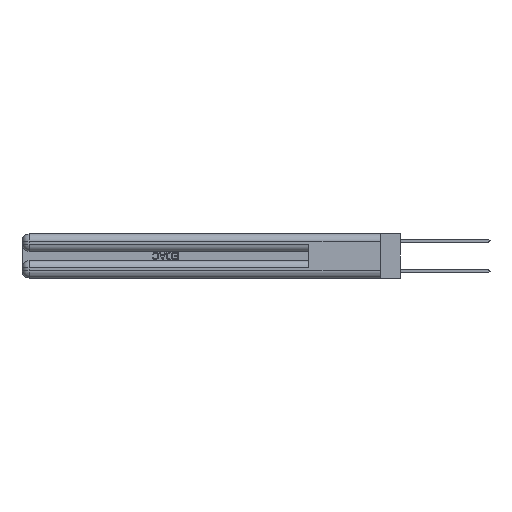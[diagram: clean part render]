
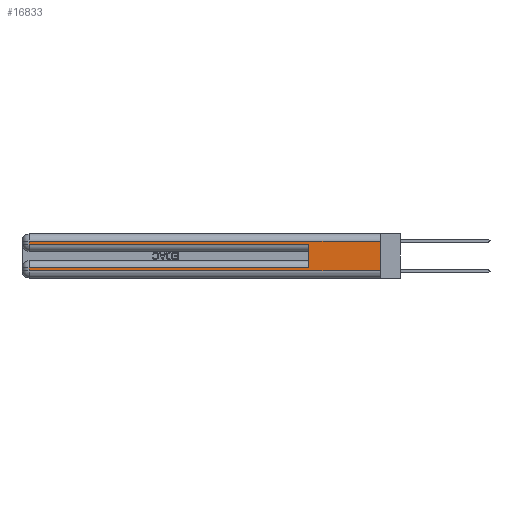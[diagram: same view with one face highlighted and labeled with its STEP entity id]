
A CAD part, left-side view. The second image highlights one B-rep face of the part: STEP entity #16833.
In plain terms, the highlighted planar face has unit normal (-1, 0, 0).
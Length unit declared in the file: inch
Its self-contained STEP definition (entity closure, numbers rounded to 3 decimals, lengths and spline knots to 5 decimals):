
#198 = EDGE_CURVE ( 'NONE', #7042, #27599, #11728, .T. ) ;
#720 = ORIENTED_EDGE ( 'NONE', *, *, #17180, .F. ) ;
#1212 = CARTESIAN_POINT ( 'NONE',  ( 0., 0.6, 0.285 ) ) ;
#1378 = CARTESIAN_POINT ( 'NONE',  ( 0., 0., 0.285 ) ) ;
#2588 = ORIENTED_EDGE ( 'NONE', *, *, #14866, .T. ) ;
#3160 = ORIENTED_EDGE ( 'NONE', *, *, #25296, .F. ) ;
#3190 = CARTESIAN_POINT ( 'NONE',  ( 0., 0., 0.37 ) ) ;
#4592 = EDGE_CURVE ( 'NONE', #10949, #34986, #30109, .T. ) ;
#5843 = CARTESIAN_POINT ( 'NONE',  ( 0., 0., 0.06 ) ) ;
#5926 = DIRECTION ( 'NONE',  ( 0., 0., 1. ) ) ;
#6477 = CARTESIAN_POINT ( 'NONE',  ( 0., 0., 0.31 ) ) ;
#6517 = FACE_OUTER_BOUND ( 'NONE', #27968, .T. ) ;
#7042 = VERTEX_POINT ( 'NONE', #21758 ) ;
#7309 = CARTESIAN_POINT ( 'NONE',  ( 0., 2.94, 0.06 ) ) ;
#7376 = VERTEX_POINT ( 'NONE', #7309 ) ;
#7793 = DIRECTION ( 'NONE',  ( 0., 0., -1. ) ) ;
#7991 = CARTESIAN_POINT ( 'NONE',  ( 0., 0., 0.37 ) ) ;
#8673 = LINE ( 'NONE', #25669, #31384 ) ;
#9065 = CARTESIAN_POINT ( 'NONE',  ( 0., 2.94, 0.085 ) ) ;
#10949 = VERTEX_POINT ( 'NONE', #22416 ) ;
#11449 = LINE ( 'NONE', #5843, #21288 ) ;
#11728 = LINE ( 'NONE', #6477, #22812 ) ;
#11773 = PLANE ( 'NONE',  #25921 ) ;
#11873 = VECTOR ( 'NONE', #5926, 39.37008 ) ;
#13426 = LINE ( 'NONE', #7991, #13972 ) ;
#13459 = EDGE_CURVE ( 'NONE', #27599, #10949, #15153, .T. ) ;
#13959 = LINE ( 'NONE', #25172, #11873 ) ;
#13972 = VECTOR ( 'NONE', #7793, 39.37008 ) ;
#14409 = VERTEX_POINT ( 'NONE', #9065 ) ;
#14560 = DIRECTION ( 'NONE',  ( 1., 0., 0. ) ) ;
#14866 = EDGE_CURVE ( 'NONE', #14409, #7376, #17289, .T. ) ;
#15142 = CARTESIAN_POINT ( 'NONE',  ( 0., 2.94, 0.31 ) ) ;
#15153 = LINE ( 'NONE', #35053, #28697 ) ;
#15573 = CARTESIAN_POINT ( 'NONE',  ( 0., 0., 0.06 ) ) ;
#16241 = ORIENTED_EDGE ( 'NONE', *, *, #13459, .T. ) ;
#16833 = ADVANCED_FACE ( 'NONE', ( #6517 ), #11773, .F. ) ;
#17180 = EDGE_CURVE ( 'NONE', #7042, #26058, #13426, .T. ) ;
#17289 = LINE ( 'NONE', #28630, #29357 ) ;
#19382 = VERTEX_POINT ( 'NONE', #27951 ) ;
#21129 = DIRECTION ( 'NONE',  ( 0., 0., -1. ) ) ;
#21272 = EDGE_CURVE ( 'NONE', #19382, #14409, #8673, .T. ) ;
#21288 = VECTOR ( 'NONE', #34528, 39.37008 ) ;
#21702 = EDGE_CURVE ( 'NONE', #7376, #26058, #11449, .T. ) ;
#21758 = CARTESIAN_POINT ( 'NONE',  ( 0., 0., 0.31 ) ) ;
#22330 = ORIENTED_EDGE ( 'NONE', *, *, #4592, .T. ) ;
#22416 = CARTESIAN_POINT ( 'NONE',  ( 0., 2.94, 0.285 ) ) ;
#22812 = VECTOR ( 'NONE', #34435, 39.37008 ) ;
#24025 = ORIENTED_EDGE ( 'NONE', *, *, #198, .T. ) ;
#25172 = CARTESIAN_POINT ( 'NONE',  ( 0., 0.6, 0.145 ) ) ;
#25296 = EDGE_CURVE ( 'NONE', #19382, #34986, #13959, .T. ) ;
#25669 = CARTESIAN_POINT ( 'NONE',  ( 0., 0., 0.085 ) ) ;
#25921 = AXIS2_PLACEMENT_3D ( 'NONE', #3190, #14560, #28913 ) ;
#26058 = VERTEX_POINT ( 'NONE', #15573 ) ;
#26941 = DIRECTION ( 'NONE',  ( 0., -1., 0. ) ) ;
#27599 = VERTEX_POINT ( 'NONE', #15142 ) ;
#27951 = CARTESIAN_POINT ( 'NONE',  ( 0., 0.6, 0.085 ) ) ;
#27968 = EDGE_LOOP ( 'NONE', ( #720, #24025, #16241, #22330, #3160, #36279, #2588, #36660 ) ) ;
#28614 = VECTOR ( 'NONE', #26941, 39.37008 ) ;
#28630 = CARTESIAN_POINT ( 'NONE',  ( 0., 2.94, 0.37 ) ) ;
#28697 = VECTOR ( 'NONE', #21129, 39.37008 ) ;
#28913 = DIRECTION ( 'NONE',  ( 0., 0., -1. ) ) ;
#29357 = VECTOR ( 'NONE', #31960, 39.37008 ) ;
#30109 = LINE ( 'NONE', #1378, #28614 ) ;
#31384 = VECTOR ( 'NONE', #33524, 39.37008 ) ;
#31960 = DIRECTION ( 'NONE',  ( 0., 0., -1. ) ) ;
#33524 = DIRECTION ( 'NONE',  ( 0., 1., 0. ) ) ;
#34435 = DIRECTION ( 'NONE',  ( 0., 1., 0. ) ) ;
#34528 = DIRECTION ( 'NONE',  ( 0., -1., 0. ) ) ;
#34986 = VERTEX_POINT ( 'NONE', #1212 ) ;
#35053 = CARTESIAN_POINT ( 'NONE',  ( 0., 2.94, 0.37 ) ) ;
#36279 = ORIENTED_EDGE ( 'NONE', *, *, #21272, .T. ) ;
#36660 = ORIENTED_EDGE ( 'NONE', *, *, #21702, .T. ) ;
